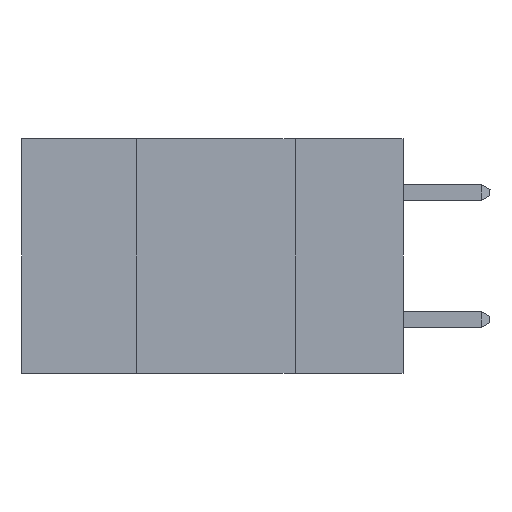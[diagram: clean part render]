
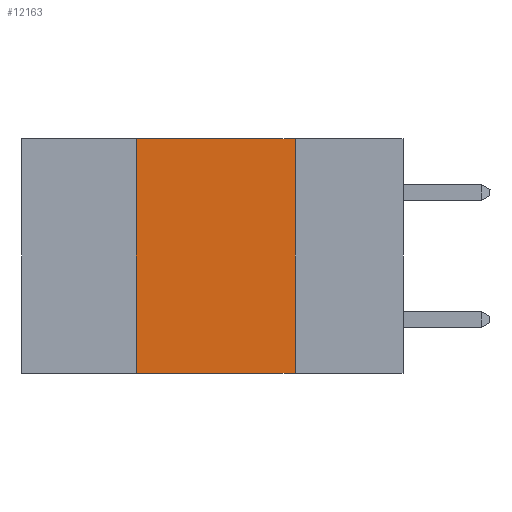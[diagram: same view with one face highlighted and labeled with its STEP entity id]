
A CAD part, left-side view. The second image highlights one B-rep face of the part: STEP entity #12163.
In plain terms, the highlighted planar face has unit normal (-1, 0, 0).
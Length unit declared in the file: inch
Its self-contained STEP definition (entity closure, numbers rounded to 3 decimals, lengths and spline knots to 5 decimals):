
#50 = LINE ( 'NONE', #16315, #1470 ) ;
#476 = DIRECTION ( 'NONE',  ( 0., -1., 0. ) ) ;
#1369 = LINE ( 'NONE', #14051, #9143 ) ;
#1470 = VECTOR ( 'NONE', #476, 39.37008 ) ;
#1723 = DIRECTION ( 'NONE',  ( 0., 0., -1. ) ) ;
#1897 = CARTESIAN_POINT ( 'NONE',  ( 0., 0.6, 0. ) ) ;
#1955 = VECTOR ( 'NONE', #16228, 39.37008 ) ;
#2072 = EDGE_CURVE ( 'NONE', #5687, #9791, #1369, .T. ) ;
#2394 = ORIENTED_EDGE ( 'NONE', *, *, #13634, .F. ) ;
#4663 = VECTOR ( 'NONE', #9452, 39.37008 ) ;
#5041 = VERTEX_POINT ( 'NONE', #11134 ) ;
#5687 = VERTEX_POINT ( 'NONE', #7009 ) ;
#5804 = PLANE ( 'NONE',  #8466 ) ;
#6232 = DIRECTION ( 'NONE',  ( 0., -1., 0. ) ) ;
#6848 = LINE ( 'NONE', #8381, #1955 ) ;
#6885 = DIRECTION ( 'NONE',  ( 1., 0., 0. ) ) ;
#7009 = CARTESIAN_POINT ( 'NONE',  ( 0., 0.42, -0.37 ) ) ;
#8100 = CARTESIAN_POINT ( 'NONE',  ( 0., 0.42, 0. ) ) ;
#8153 = LINE ( 'NONE', #8100, #4663 ) ;
#8381 = CARTESIAN_POINT ( 'NONE',  ( 0., 0.17, 0. ) ) ;
#8466 = AXIS2_PLACEMENT_3D ( 'NONE', #1897, #6885, #1723 ) ;
#9143 = VECTOR ( 'NONE', #6232, 39.37008 ) ;
#9452 = DIRECTION ( 'NONE',  ( 0., 0., 1. ) ) ;
#9791 = VERTEX_POINT ( 'NONE', #14035 ) ;
#10898 = EDGE_CURVE ( 'NONE', #5041, #16687, #50, .T. ) ;
#11134 = CARTESIAN_POINT ( 'NONE',  ( 0., 0.42, 0. ) ) ;
#11392 = FACE_OUTER_BOUND ( 'NONE', #13018, .T. ) ;
#11473 = EDGE_CURVE ( 'NONE', #5687, #5041, #8153, .T. ) ;
#12163 = ADVANCED_FACE ( 'NONE', ( #11392 ), #5804, .F. ) ;
#12789 = ORIENTED_EDGE ( 'NONE', *, *, #11473, .F. ) ;
#12931 = CARTESIAN_POINT ( 'NONE',  ( 0., 0.17, 0. ) ) ;
#13018 = EDGE_LOOP ( 'NONE', ( #2394, #16622, #12789, #14653 ) ) ;
#13634 = EDGE_CURVE ( 'NONE', #16687, #9791, #6848, .T. ) ;
#14035 = CARTESIAN_POINT ( 'NONE',  ( 0., 0.17, -0.37 ) ) ;
#14051 = CARTESIAN_POINT ( 'NONE',  ( 0., 0.6, -0.37 ) ) ;
#14653 = ORIENTED_EDGE ( 'NONE', *, *, #2072, .T. ) ;
#16228 = DIRECTION ( 'NONE',  ( 0., 0., -1. ) ) ;
#16315 = CARTESIAN_POINT ( 'NONE',  ( 0., 0.6, 0. ) ) ;
#16622 = ORIENTED_EDGE ( 'NONE', *, *, #10898, .F. ) ;
#16687 = VERTEX_POINT ( 'NONE', #12931 ) ;
